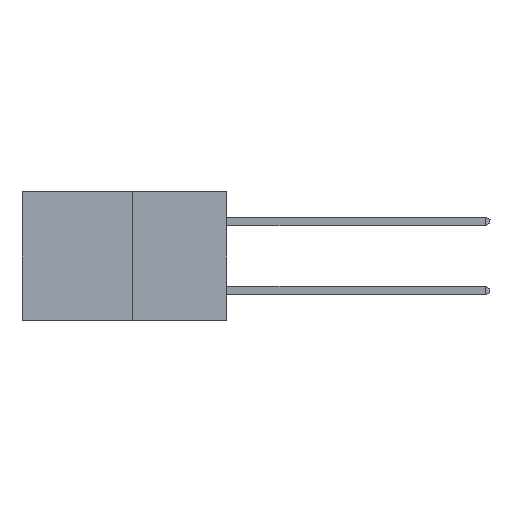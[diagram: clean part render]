
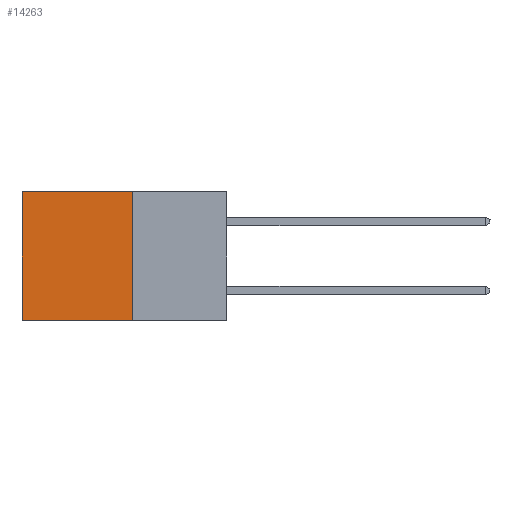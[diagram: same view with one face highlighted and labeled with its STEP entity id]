
A CAD part, left-side view. The second image highlights one B-rep face of the part: STEP entity #14263.
In plain terms, the highlighted planar face has unit normal (-1, 0, 0).
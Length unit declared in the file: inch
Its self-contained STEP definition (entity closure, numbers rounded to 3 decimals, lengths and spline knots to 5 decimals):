
#1108 = DIRECTION ( 'NONE',  ( 0., 0., -1. ) ) ;
#1431 = VERTEX_POINT ( 'NONE', #1784 ) ;
#1551 = LINE ( 'NONE', #8994, #4531 ) ;
#1747 = CARTESIAN_POINT ( 'NONE',  ( 0.277, 0.27, -0.37 ) ) ;
#1750 = VERTEX_POINT ( 'NONE', #15330 ) ;
#1784 = CARTESIAN_POINT ( 'NONE',  ( 0.277, 0.59, 0. ) ) ;
#2135 = LINE ( 'NONE', #15548, #5509 ) ;
#2248 = ORIENTED_EDGE ( 'NONE', *, *, #3174, .F. ) ;
#3174 = EDGE_CURVE ( 'NONE', #13286, #4237, #1551, .T. ) ;
#3220 = DIRECTION ( 'NONE',  ( 0., 1., 0. ) ) ;
#3800 = EDGE_CURVE ( 'NONE', #1431, #4237, #2135, .T. ) ;
#4237 = VERTEX_POINT ( 'NONE', #9610 ) ;
#4531 = VECTOR ( 'NONE', #3220, 39.37008 ) ;
#5509 = VECTOR ( 'NONE', #15176, 39.37008 ) ;
#5526 = EDGE_CURVE ( 'NONE', #1750, #13286, #12754, .T. ) ;
#6406 = ORIENTED_EDGE ( 'NONE', *, *, #5526, .F. ) ;
#6974 = CARTESIAN_POINT ( 'NONE',  ( 0.277, 0.27, 0. ) ) ;
#7035 = LINE ( 'NONE', #6974, #10857 ) ;
#7444 = PLANE ( 'NONE',  #12368 ) ;
#7861 = ORIENTED_EDGE ( 'NONE', *, *, #13354, .T. ) ;
#7870 = EDGE_LOOP ( 'NONE', ( #8442, #2248, #6406, #7861 ) ) ;
#8442 = ORIENTED_EDGE ( 'NONE', *, *, #3800, .T. ) ;
#8778 = DIRECTION ( 'NONE',  ( 1., 0., 0. ) ) ;
#8994 = CARTESIAN_POINT ( 'NONE',  ( 0.277, 0.27, -0.37 ) ) ;
#9235 = DIRECTION ( 'NONE',  ( 0., 0., -1. ) ) ;
#9610 = CARTESIAN_POINT ( 'NONE',  ( 0.277, 0.59, -0.37 ) ) ;
#9976 = CARTESIAN_POINT ( 'NONE',  ( 0.277, 0.27, -0.37 ) ) ;
#10857 = VECTOR ( 'NONE', #15524, 39.37008 ) ;
#12038 = VECTOR ( 'NONE', #9235, 39.37008 ) ;
#12368 = AXIS2_PLACEMENT_3D ( 'NONE', #15946, #8778, #1108 ) ;
#12754 = LINE ( 'NONE', #9976, #12038 ) ;
#12854 = FACE_OUTER_BOUND ( 'NONE', #7870, .T. ) ;
#13286 = VERTEX_POINT ( 'NONE', #1747 ) ;
#13354 = EDGE_CURVE ( 'NONE', #1750, #1431, #7035, .T. ) ;
#14263 = ADVANCED_FACE ( 'NONE', ( #12854 ), #7444, .F. ) ;
#15176 = DIRECTION ( 'NONE',  ( 0., 0., -1. ) ) ;
#15330 = CARTESIAN_POINT ( 'NONE',  ( 0.277, 0.27, 0. ) ) ;
#15524 = DIRECTION ( 'NONE',  ( 0., 1., 0. ) ) ;
#15548 = CARTESIAN_POINT ( 'NONE',  ( 0.277, 0.59, -0.37 ) ) ;
#15946 = CARTESIAN_POINT ( 'NONE',  ( 0.277, 0.27, -0.37 ) ) ;
